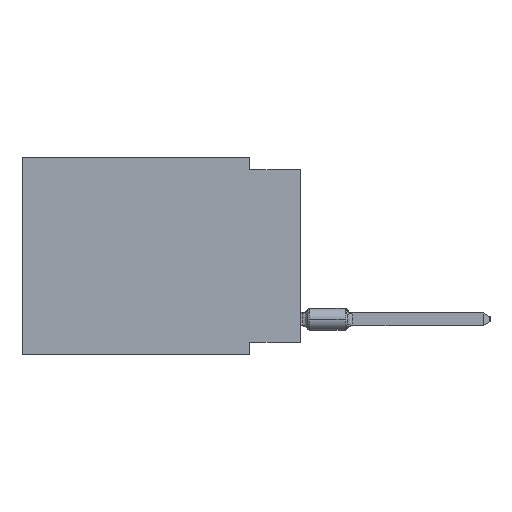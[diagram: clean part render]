
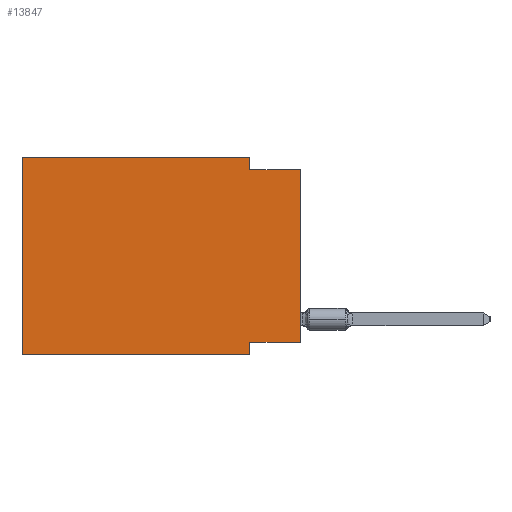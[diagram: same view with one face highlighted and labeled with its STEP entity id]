
A CAD part, left-side view. The second image highlights one B-rep face of the part: STEP entity #13847.
In plain terms, the highlighted planar face has unit normal (-1, 0, 0).
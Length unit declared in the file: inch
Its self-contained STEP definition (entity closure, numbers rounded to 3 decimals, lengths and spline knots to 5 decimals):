
#576 = LINE ( 'NONE', #59283, #44373 ) ;
#2224 = EDGE_CURVE ( 'NONE', #20492, #26911, #27133, .T. ) ;
#2534 = EDGE_CURVE ( 'NONE', #39835, #28639, #52216, .T. ) ;
#5334 = ORIENTED_EDGE ( 'NONE', *, *, #22661, .F. ) ;
#7459 = AXIS2_PLACEMENT_3D ( 'NONE', #42417, #32451, #22107 ) ;
#8094 = VERTEX_POINT ( 'NONE', #68486 ) ;
#11005 = VECTOR ( 'NONE', #46342, 39.37008 ) ;
#12758 = ORIENTED_EDGE ( 'NONE', *, *, #31281, .F. ) ;
#13241 = CARTESIAN_POINT ( 'NONE',  ( 0., 0.1, -0.39 ) ) ;
#13411 = LINE ( 'NONE', #62509, #38020 ) ;
#13847 = ADVANCED_FACE ( 'NONE', ( #14688 ), #49163, .F. ) ;
#14688 = FACE_OUTER_BOUND ( 'NONE', #43496, .T. ) ;
#15204 = VECTOR ( 'NONE', #19460, 39.37008 ) ;
#17256 = CARTESIAN_POINT ( 'NONE',  ( 0., 0.55, 0. ) ) ;
#17699 = DIRECTION ( 'NONE',  ( 0., 0., 1. ) ) ;
#18417 = LINE ( 'NONE', #23393, #42842 ) ;
#19460 = DIRECTION ( 'NONE',  ( 0., -1., 0. ) ) ;
#19615 = DIRECTION ( 'NONE',  ( 0., 0., -1. ) ) ;
#20492 = VERTEX_POINT ( 'NONE', #23414 ) ;
#21083 = ORIENTED_EDGE ( 'NONE', *, *, #58838, .F. ) ;
#21275 = ORIENTED_EDGE ( 'NONE', *, *, #23793, .T. ) ;
#22107 = DIRECTION ( 'NONE',  ( 0., 0., -1. ) ) ;
#22661 = EDGE_CURVE ( 'NONE', #28639, #35247, #30313, .T. ) ;
#23393 = CARTESIAN_POINT ( 'NONE',  ( 0., 0., 0. ) ) ;
#23414 = CARTESIAN_POINT ( 'NONE',  ( 0., 0., -0.365 ) ) ;
#23793 = EDGE_CURVE ( 'NONE', #30552, #8094, #576, .T. ) ;
#24611 = CARTESIAN_POINT ( 'NONE',  ( 0., 0.1, 0. ) ) ;
#26514 = CARTESIAN_POINT ( 'NONE',  ( 0., 0.55, -0.39 ) ) ;
#26911 = VERTEX_POINT ( 'NONE', #44852 ) ;
#27133 = LINE ( 'NONE', #27470, #68634 ) ;
#27470 = CARTESIAN_POINT ( 'NONE',  ( 0., 0., -0.365 ) ) ;
#28190 = DIRECTION ( 'NONE',  ( 0., 1., 0. ) ) ;
#28639 = VERTEX_POINT ( 'NONE', #45831 ) ;
#30313 = LINE ( 'NONE', #24611, #43052 ) ;
#30552 = VERTEX_POINT ( 'NONE', #26514 ) ;
#30726 = VECTOR ( 'NONE', #49650, 39.37008 ) ;
#31281 = EDGE_CURVE ( 'NONE', #26911, #8094, #66983, .T. ) ;
#32044 = EDGE_CURVE ( 'NONE', #20492, #59182, #18417, .T. ) ;
#32451 = DIRECTION ( 'NONE',  ( 1., 0., 0. ) ) ;
#33024 = ORIENTED_EDGE ( 'NONE', *, *, #2224, .F. ) ;
#33844 = ORIENTED_EDGE ( 'NONE', *, *, #32044, .T. ) ;
#35247 = VERTEX_POINT ( 'NONE', #53485 ) ;
#38020 = VECTOR ( 'NONE', #49821, 39.37008 ) ;
#39692 = LINE ( 'NONE', #17256, #30726 ) ;
#39835 = VERTEX_POINT ( 'NONE', #67418 ) ;
#42417 = CARTESIAN_POINT ( 'NONE',  ( 0., 0.55, 0. ) ) ;
#42842 = VECTOR ( 'NONE', #17699, 39.37008 ) ;
#43052 = VECTOR ( 'NONE', #19615, 39.37008 ) ;
#43496 = EDGE_LOOP ( 'NONE', ( #33844, #44049, #5334, #48519, #21083, #21275, #12758, #33024 ) ) ;
#44049 = ORIENTED_EDGE ( 'NONE', *, *, #65124, .F. ) ;
#44319 = DIRECTION ( 'NONE',  ( 0., -1., 0. ) ) ;
#44373 = VECTOR ( 'NONE', #44319, 39.37008 ) ;
#44852 = CARTESIAN_POINT ( 'NONE',  ( 0., 0.1, -0.365 ) ) ;
#45831 = CARTESIAN_POINT ( 'NONE',  ( 0., 0.1, 0. ) ) ;
#46342 = DIRECTION ( 'NONE',  ( 0., 0., -1. ) ) ;
#48519 = ORIENTED_EDGE ( 'NONE', *, *, #2534, .F. ) ;
#49163 = PLANE ( 'NONE',  #7459 ) ;
#49650 = DIRECTION ( 'NONE',  ( 0., 0., 1. ) ) ;
#49821 = DIRECTION ( 'NONE',  ( 0., -1., 0. ) ) ;
#52216 = LINE ( 'NONE', #61834, #15204 ) ;
#53485 = CARTESIAN_POINT ( 'NONE',  ( 0., 0.1, -0.025 ) ) ;
#58838 = EDGE_CURVE ( 'NONE', #30552, #39835, #39692, .T. ) ;
#58851 = CARTESIAN_POINT ( 'NONE',  ( 0., 0., -0.025 ) ) ;
#59182 = VERTEX_POINT ( 'NONE', #58851 ) ;
#59283 = CARTESIAN_POINT ( 'NONE',  ( 0., 0.55, -0.39 ) ) ;
#61834 = CARTESIAN_POINT ( 'NONE',  ( 0., 0.55, 0. ) ) ;
#62509 = CARTESIAN_POINT ( 'NONE',  ( 0., 0., -0.025 ) ) ;
#65124 = EDGE_CURVE ( 'NONE', #35247, #59182, #13411, .T. ) ;
#66983 = LINE ( 'NONE', #13241, #11005 ) ;
#67418 = CARTESIAN_POINT ( 'NONE',  ( 0., 0.55, 0. ) ) ;
#68486 = CARTESIAN_POINT ( 'NONE',  ( 0., 0.1, -0.39 ) ) ;
#68634 = VECTOR ( 'NONE', #28190, 39.37008 ) ;
